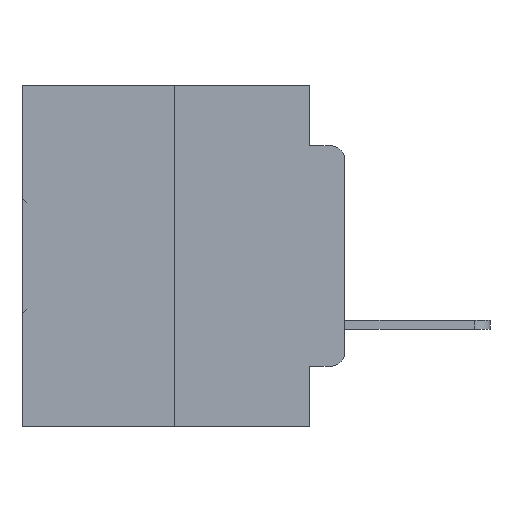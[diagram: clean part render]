
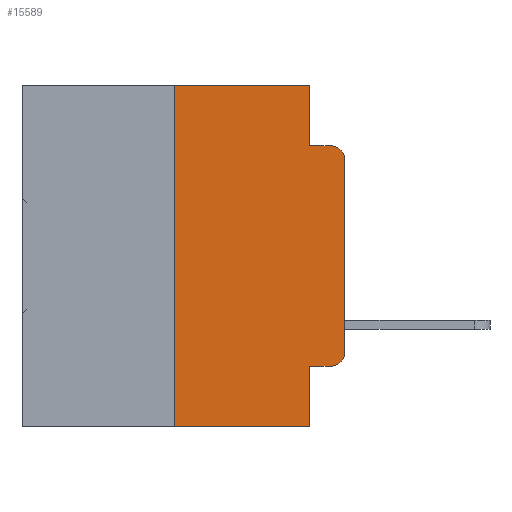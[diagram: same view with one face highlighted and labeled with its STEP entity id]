
A CAD part, left-side view. The second image highlights one B-rep face of the part: STEP entity #15589.
In plain terms, the highlighted planar face has unit normal (-1, 0, 0).
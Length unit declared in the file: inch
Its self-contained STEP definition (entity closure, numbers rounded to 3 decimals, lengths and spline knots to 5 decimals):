
#63 = DIRECTION ( 'NONE',  ( 0., 0., -1. ) ) ;
#485 = VERTEX_POINT ( 'NONE', #11925 ) ;
#1224 = CARTESIAN_POINT ( 'NONE',  ( 0., 0.051, 0. ) ) ;
#1378 = EDGE_CURVE ( 'NONE', #25823, #485, #20427, .T. ) ;
#1827 = ORIENTED_EDGE ( 'NONE', *, *, #23055, .T. ) ;
#2679 = CARTESIAN_POINT ( 'NONE',  ( 0., 0.473, -0.5 ) ) ;
#2760 = ORIENTED_EDGE ( 'NONE', *, *, #26238, .F. ) ;
#3218 = VECTOR ( 'NONE', #31620, 39.37008 ) ;
#3381 = ORIENTED_EDGE ( 'NONE', *, *, #1378, .T. ) ;
#3447 = VERTEX_POINT ( 'NONE', #5953 ) ;
#3557 = DIRECTION ( 'NONE',  ( 0., -1., 0. ) ) ;
#3996 = CARTESIAN_POINT ( 'NONE',  ( 0., 0.02, -0.1085 ) ) ;
#4014 = LINE ( 'NONE', #26936, #3218 ) ;
#4125 = CARTESIAN_POINT ( 'NONE',  ( 0., 0., -0.3915 ) ) ;
#4375 = ORIENTED_EDGE ( 'NONE', *, *, #24662, .T. ) ;
#4699 = VERTEX_POINT ( 'NONE', #21637 ) ;
#5467 = CARTESIAN_POINT ( 'NONE',  ( 0., 0.051, -0.4115 ) ) ;
#5553 = CARTESIAN_POINT ( 'NONE',  ( 0., 0.25, 0. ) ) ;
#5860 = VECTOR ( 'NONE', #63, 39.37008 ) ;
#5953 = CARTESIAN_POINT ( 'NONE',  ( 0., 0.02, -0.0885 ) ) ;
#6333 = LINE ( 'NONE', #11025, #31469 ) ;
#6648 = DIRECTION ( 'NONE',  ( 0., 0., -1. ) ) ;
#6744 = CARTESIAN_POINT ( 'NONE',  ( 0., 0.02, -0.3915 ) ) ;
#8052 = CIRCLE ( 'NONE', #10677, 0.02 ) ;
#9150 = DIRECTION ( 'NONE',  ( 0., 0., -1. ) ) ;
#9300 = DIRECTION ( 'NONE',  ( 0., 0., -1. ) ) ;
#9660 = ORIENTED_EDGE ( 'NONE', *, *, #22724, .F. ) ;
#10093 = VECTOR ( 'NONE', #10908, 39.37008 ) ;
#10129 = DIRECTION ( 'NONE',  ( 1., 0., 0. ) ) ;
#10677 = AXIS2_PLACEMENT_3D ( 'NONE', #6744, #24076, #9300 ) ;
#10896 = EDGE_CURVE ( 'NONE', #14277, #3447, #28746, .T. ) ;
#10908 = DIRECTION ( 'NONE',  ( 0., -1., 0. ) ) ;
#11025 = CARTESIAN_POINT ( 'NONE',  ( 0., 0., 0. ) ) ;
#11117 = DIRECTION ( 'NONE',  ( 0., 0., 1. ) ) ;
#11925 = CARTESIAN_POINT ( 'NONE',  ( 0., 0.051, -0.5 ) ) ;
#12069 = VECTOR ( 'NONE', #15732, 39.37008 ) ;
#13144 = LINE ( 'NONE', #1224, #24625 ) ;
#14230 = EDGE_CURVE ( 'NONE', #28180, #3447, #16386, .T. ) ;
#14252 = VERTEX_POINT ( 'NONE', #4125 ) ;
#14277 = VERTEX_POINT ( 'NONE', #26432 ) ;
#14647 = VECTOR ( 'NONE', #3557, 39.37008 ) ;
#15061 = VERTEX_POINT ( 'NONE', #25385 ) ;
#15297 = ORIENTED_EDGE ( 'NONE', *, *, #30942, .F. ) ;
#15589 = ADVANCED_FACE ( 'NONE', ( #19735 ), #29464, .F. ) ;
#15732 = DIRECTION ( 'NONE',  ( 0., 0., 1. ) ) ;
#16386 = CIRCLE ( 'NONE', #28471, 0.02 ) ;
#16752 = AXIS2_PLACEMENT_3D ( 'NONE', #20008, #10129, #27209 ) ;
#17617 = EDGE_CURVE ( 'NONE', #14252, #28180, #6333, .T. ) ;
#18022 = DIRECTION ( 'NONE',  ( 0., -1., 0. ) ) ;
#18226 = ORIENTED_EDGE ( 'NONE', *, *, #10896, .F. ) ;
#18384 = CARTESIAN_POINT ( 'NONE',  ( 0., 0.051, 0. ) ) ;
#19735 = FACE_OUTER_BOUND ( 'NONE', #28664, .T. ) ;
#20008 = CARTESIAN_POINT ( 'NONE',  ( 0., 0.473, 0. ) ) ;
#20230 = CARTESIAN_POINT ( 'NONE',  ( 0., 0.02, -0.4115 ) ) ;
#20427 = LINE ( 'NONE', #2679, #14647 ) ;
#20522 = CARTESIAN_POINT ( 'NONE',  ( 0., 0.051, 0. ) ) ;
#21532 = ORIENTED_EDGE ( 'NONE', *, *, #27809, .F. ) ;
#21541 = DIRECTION ( 'NONE',  ( -1., 0., 0. ) ) ;
#21637 = CARTESIAN_POINT ( 'NONE',  ( 0., 0.25, 0. ) ) ;
#22381 = CARTESIAN_POINT ( 'NONE',  ( 0., 0.25, -0.5 ) ) ;
#22724 = EDGE_CURVE ( 'NONE', #4699, #27023, #4014, .T. ) ;
#23055 = EDGE_CURVE ( 'NONE', #31252, #14252, #8052, .T. ) ;
#24032 = ORIENTED_EDGE ( 'NONE', *, *, #14230, .T. ) ;
#24076 = DIRECTION ( 'NONE',  ( -1., 0., 0. ) ) ;
#24625 = VECTOR ( 'NONE', #9150, 39.37008 ) ;
#24662 = EDGE_CURVE ( 'NONE', #15061, #31252, #30081, .T. ) ;
#25385 = CARTESIAN_POINT ( 'NONE',  ( 0., 0.051, -0.4115 ) ) ;
#25569 = LINE ( 'NONE', #20522, #5860 ) ;
#25823 = VERTEX_POINT ( 'NONE', #22381 ) ;
#26238 = EDGE_CURVE ( 'NONE', #15061, #485, #25569, .T. ) ;
#26432 = CARTESIAN_POINT ( 'NONE',  ( 0., 0.051, -0.0885 ) ) ;
#26936 = CARTESIAN_POINT ( 'NONE',  ( 0., 0.473, 0. ) ) ;
#27023 = VERTEX_POINT ( 'NONE', #18384 ) ;
#27209 = DIRECTION ( 'NONE',  ( 0., 0., -1. ) ) ;
#27775 = ORIENTED_EDGE ( 'NONE', *, *, #17617, .T. ) ;
#27809 = EDGE_CURVE ( 'NONE', #25823, #4699, #32014, .T. ) ;
#27910 = CARTESIAN_POINT ( 'NONE',  ( 0., 0.051, -0.0885 ) ) ;
#28180 = VERTEX_POINT ( 'NONE', #28993 ) ;
#28471 = AXIS2_PLACEMENT_3D ( 'NONE', #3996, #21541, #6648 ) ;
#28590 = VECTOR ( 'NONE', #18022, 39.37008 ) ;
#28664 = EDGE_LOOP ( 'NONE', ( #27775, #24032, #18226, #15297, #9660, #21532, #3381, #2760, #4375, #1827 ) ) ;
#28746 = LINE ( 'NONE', #27910, #10093 ) ;
#28993 = CARTESIAN_POINT ( 'NONE',  ( 0., 0., -0.1085 ) ) ;
#29464 = PLANE ( 'NONE',  #16752 ) ;
#30081 = LINE ( 'NONE', #5467, #28590 ) ;
#30942 = EDGE_CURVE ( 'NONE', #27023, #14277, #13144, .T. ) ;
#31252 = VERTEX_POINT ( 'NONE', #20230 ) ;
#31469 = VECTOR ( 'NONE', #11117, 39.37008 ) ;
#31620 = DIRECTION ( 'NONE',  ( 0., -1., 0. ) ) ;
#32014 = LINE ( 'NONE', #5553, #12069 ) ;
